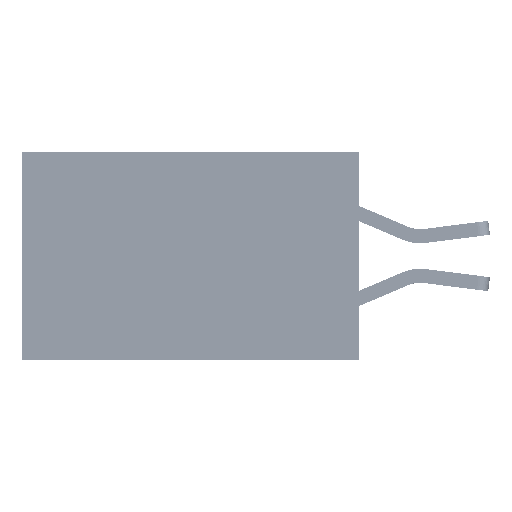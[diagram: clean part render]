
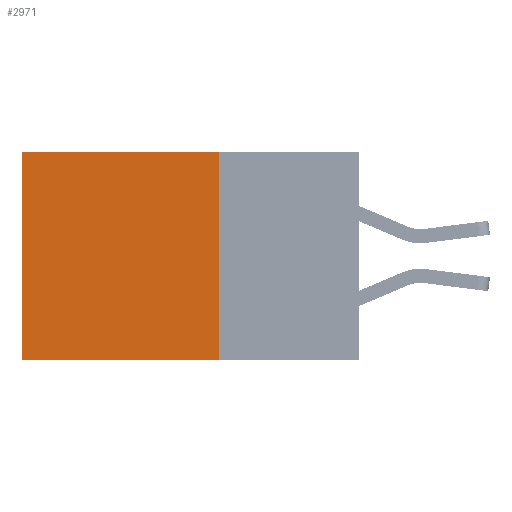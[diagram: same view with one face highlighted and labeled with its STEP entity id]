
A CAD part, left-side view. The second image highlights one B-rep face of the part: STEP entity #2971.
In plain terms, the highlighted planar face has unit normal (-1, 0, 0).
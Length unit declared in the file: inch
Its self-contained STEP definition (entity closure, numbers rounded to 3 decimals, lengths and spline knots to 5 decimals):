
#790 = EDGE_CURVE ( 'NONE', #40160, #3785, #42813, .T. ) ;
#2971 = ADVANCED_FACE ( 'NONE', ( #19198 ), #45259, .F. ) ;
#3785 = VERTEX_POINT ( 'NONE', #22316 ) ;
#4405 = LINE ( 'NONE', #28454, #25061 ) ;
#5482 = VECTOR ( 'NONE', #49359, 39.37008 ) ;
#12993 = EDGE_LOOP ( 'NONE', ( #35317, #41476, #36058, #45096 ) ) ;
#13230 = DIRECTION ( 'NONE',  ( 1., 0., 0. ) ) ;
#14779 = LINE ( 'NONE', #22349, #45797 ) ;
#19198 = FACE_OUTER_BOUND ( 'NONE', #12993, .T. ) ;
#19490 = CARTESIAN_POINT ( 'NONE',  ( 0.2875, 0.25, -0.37 ) ) ;
#22316 = CARTESIAN_POINT ( 'NONE',  ( 0.2875, 0.6, -0.37 ) ) ;
#22349 = CARTESIAN_POINT ( 'NONE',  ( 0.2875, 0.6, 0. ) ) ;
#22803 = CARTESIAN_POINT ( 'NONE',  ( 0.2875, 0.6, 0. ) ) ;
#25061 = VECTOR ( 'NONE', #32509, 39.37008 ) ;
#26289 = EDGE_CURVE ( 'NONE', #39364, #40160, #4405, .T. ) ;
#26450 = DIRECTION ( 'NONE',  ( 0., 0., -1. ) ) ;
#28454 = CARTESIAN_POINT ( 'NONE',  ( 0.2875, 0.25, 0. ) ) ;
#28467 = EDGE_CURVE ( 'NONE', #39364, #52589, #38028, .T. ) ;
#29407 = EDGE_CURVE ( 'NONE', #52589, #3785, #14779, .T. ) ;
#31784 = DIRECTION ( 'NONE',  ( 0., 1., 0. ) ) ;
#32168 = VECTOR ( 'NONE', #31784, 39.37008 ) ;
#32509 = DIRECTION ( 'NONE',  ( 0., 0., -1. ) ) ;
#34955 = CARTESIAN_POINT ( 'NONE',  ( 0.2875, 0.25, 0. ) ) ;
#35317 = ORIENTED_EDGE ( 'NONE', *, *, #29407, .T. ) ;
#36058 = ORIENTED_EDGE ( 'NONE', *, *, #26289, .F. ) ;
#38028 = LINE ( 'NONE', #45249, #5482 ) ;
#39364 = VERTEX_POINT ( 'NONE', #34955 ) ;
#40160 = VERTEX_POINT ( 'NONE', #52471 ) ;
#41476 = ORIENTED_EDGE ( 'NONE', *, *, #790, .F. ) ;
#41597 = DIRECTION ( 'NONE',  ( 0., 0., -1. ) ) ;
#42813 = LINE ( 'NONE', #19490, #32168 ) ;
#45096 = ORIENTED_EDGE ( 'NONE', *, *, #28467, .T. ) ;
#45249 = CARTESIAN_POINT ( 'NONE',  ( 0.2875, 0.25, 0. ) ) ;
#45259 = PLANE ( 'NONE',  #51878 ) ;
#45444 = CARTESIAN_POINT ( 'NONE',  ( 0.2875, 0.25, 0. ) ) ;
#45797 = VECTOR ( 'NONE', #26450, 39.37008 ) ;
#49359 = DIRECTION ( 'NONE',  ( 0., 1., 0. ) ) ;
#51878 = AXIS2_PLACEMENT_3D ( 'NONE', #45444, #13230, #41597 ) ;
#52471 = CARTESIAN_POINT ( 'NONE',  ( 0.2875, 0.25, -0.37 ) ) ;
#52589 = VERTEX_POINT ( 'NONE', #22803 ) ;
